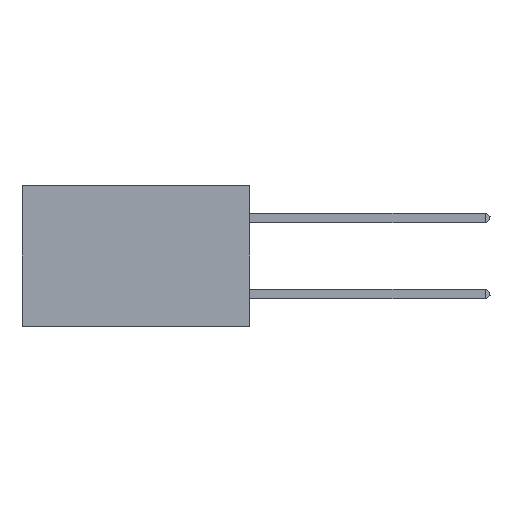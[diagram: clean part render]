
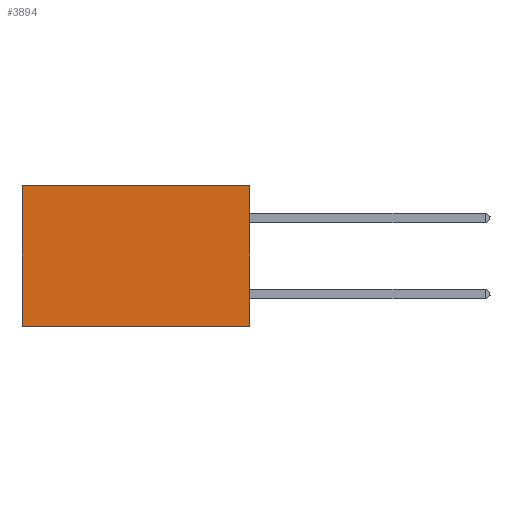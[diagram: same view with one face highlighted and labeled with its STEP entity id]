
A CAD part, left-side view. The second image highlights one B-rep face of the part: STEP entity #3894.
In plain terms, the highlighted planar face has unit normal (-1, 0, 0).
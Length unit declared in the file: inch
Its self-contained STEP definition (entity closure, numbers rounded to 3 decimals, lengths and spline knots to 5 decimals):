
#2027 = DIRECTION ( 'NONE',  ( 0., 1., 0. ) ) ;
#3715 = LINE ( 'NONE', #21759, #33691 ) ;
#3886 = PLANE ( 'NONE',  #6033 ) ;
#3894 = ADVANCED_FACE ( 'NONE', ( #20865 ), #3886, .F. ) ;
#5015 = CARTESIAN_POINT ( 'NONE',  ( 0.2875, 0., 0. ) ) ;
#6033 = AXIS2_PLACEMENT_3D ( 'NONE', #12357, #23415, #15153 ) ;
#6855 = EDGE_LOOP ( 'NONE', ( #16538, #18740, #34949, #13688 ) ) ;
#7528 = EDGE_CURVE ( 'NONE', #28467, #25957, #8319, .T. ) ;
#7979 = DIRECTION ( 'NONE',  ( 0., 1., 0. ) ) ;
#8319 = LINE ( 'NONE', #21300, #30908 ) ;
#11077 = CARTESIAN_POINT ( 'NONE',  ( 0.2875, 0.6, 0. ) ) ;
#11356 = LINE ( 'NONE', #11077, #17458 ) ;
#12357 = CARTESIAN_POINT ( 'NONE',  ( 0.2875, 0., 0. ) ) ;
#12696 = EDGE_CURVE ( 'NONE', #25957, #31206, #11356, .T. ) ;
#13688 = ORIENTED_EDGE ( 'NONE', *, *, #7528, .T. ) ;
#14429 = VERTEX_POINT ( 'NONE', #16493 ) ;
#15153 = DIRECTION ( 'NONE',  ( 0., 0., -1. ) ) ;
#16493 = CARTESIAN_POINT ( 'NONE',  ( 0.2875, 0., -0.37 ) ) ;
#16538 = ORIENTED_EDGE ( 'NONE', *, *, #12696, .T. ) ;
#17458 = VECTOR ( 'NONE', #22490, 39.37008 ) ;
#18740 = ORIENTED_EDGE ( 'NONE', *, *, #21021, .F. ) ;
#20865 = FACE_OUTER_BOUND ( 'NONE', #6855, .T. ) ;
#21021 = EDGE_CURVE ( 'NONE', #14429, #31206, #3715, .T. ) ;
#21300 = CARTESIAN_POINT ( 'NONE',  ( 0.2875, 0., 0. ) ) ;
#21759 = CARTESIAN_POINT ( 'NONE',  ( 0.2875, 0., -0.37 ) ) ;
#22490 = DIRECTION ( 'NONE',  ( 0., 0., -1. ) ) ;
#23415 = DIRECTION ( 'NONE',  ( 1., 0., 0. ) ) ;
#24888 = EDGE_CURVE ( 'NONE', #28467, #14429, #26905, .T. ) ;
#25621 = CARTESIAN_POINT ( 'NONE',  ( 0.2875, 0., 0. ) ) ;
#25957 = VERTEX_POINT ( 'NONE', #33220 ) ;
#26905 = LINE ( 'NONE', #25621, #33866 ) ;
#28467 = VERTEX_POINT ( 'NONE', #5015 ) ;
#30478 = CARTESIAN_POINT ( 'NONE',  ( 0.2875, 0.6, -0.37 ) ) ;
#30604 = DIRECTION ( 'NONE',  ( 0., 0., -1. ) ) ;
#30908 = VECTOR ( 'NONE', #2027, 39.37008 ) ;
#31206 = VERTEX_POINT ( 'NONE', #30478 ) ;
#33220 = CARTESIAN_POINT ( 'NONE',  ( 0.2875, 0.6, 0. ) ) ;
#33691 = VECTOR ( 'NONE', #7979, 39.37008 ) ;
#33866 = VECTOR ( 'NONE', #30604, 39.37008 ) ;
#34949 = ORIENTED_EDGE ( 'NONE', *, *, #24888, .F. ) ;
